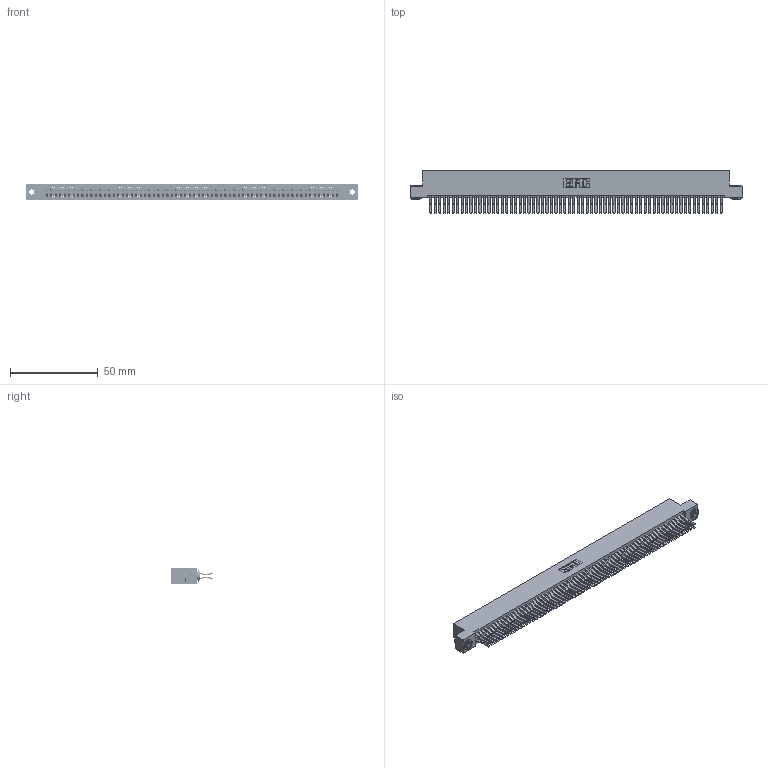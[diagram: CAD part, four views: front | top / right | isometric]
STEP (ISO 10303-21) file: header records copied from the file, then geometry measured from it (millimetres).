
FILE_DESCRIPTION (( 'STEP AP203' ), '1' );
FILE_NAME ('395-132-560-203.STEP', '2019-10-29T08:18:48', ( '' ), ( '' ), 'SwSTEP 2.0', 'SolidWorks 2016', '' );
FILE_SCHEMA (( 'CONFIG_CONTROL_DESIGN' ));
Length unit declared in the file: inch
Products named in the file (4): 345 Part_Flush Mounting Lugs - 0.156 Dia-TH; 345-292-001_560 Tail; 345-250-002_345-250-002-102; 395-132-560-203
Assembly tree (135 placements, depth 2):
  395-132-560-203
    345 Part_Flush Mounting Lugs - 0.156 Dia-TH
    345-292-001_560 Tail  x132
    345-250-002_345-250-002-102  x2
Bounding box: 188.85 x 24.45 x 9.4 mm (x, y, z)
Volume: 19452.4 mm3; surface area: 31648.8 mm2
Topology: 135 solids, 135 shells, 7028 faces, 20877 edges, 13738 vertices
Faces by surface type: plane 4446, cylinder 2574, cone 8
Entity records: 49292 total; most frequent: CARTESIAN_POINT 8215, ORIENTED_EDGE 8142, DIRECTION 7249, EDGE_CURVE 4071, LINE 3647, VECTOR 3647, VERTEX_POINT 2710, AXIS2_PLACEMENT_3D 1801
